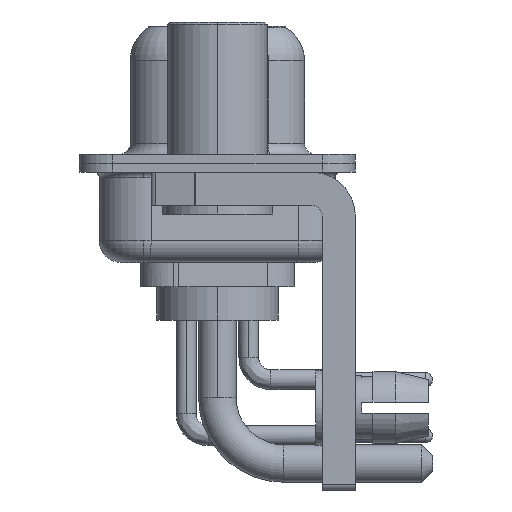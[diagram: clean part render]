
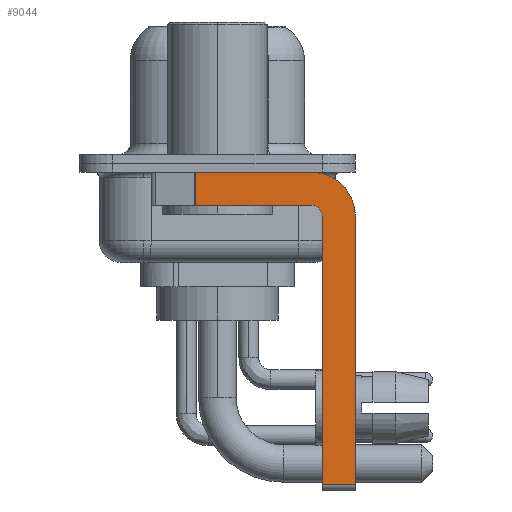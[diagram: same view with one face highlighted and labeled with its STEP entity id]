
A CAD part, left-side view. The second image highlights one B-rep face of the part: STEP entity #9044.
In plain terms, the highlighted planar face has unit normal (-1, 0, 0).
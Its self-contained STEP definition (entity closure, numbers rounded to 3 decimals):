
#429 = CARTESIAN_POINT ( 'NONE',  ( -2.9, 0.978, -0.4 ) ) ;
#444 = LINE ( 'NONE', #2135, #15913 ) ;
#1451 = EDGE_CURVE ( 'NONE', #15932, #14451, #21649, .T. ) ;
#1742 = LINE ( 'NONE', #19196, #20685 ) ;
#1947 = ORIENTED_EDGE ( 'NONE', *, *, #2216, .F. ) ;
#2135 = CARTESIAN_POINT ( 'NONE',  ( -2.9, -4.75, -14.8 ) ) ;
#2216 = EDGE_CURVE ( 'NONE', #13963, #22354, #444, .T. ) ;
#2431 = CARTESIAN_POINT ( 'NONE',  ( -2.9, 3., -0.4 ) ) ;
#3409 = ORIENTED_EDGE ( 'NONE', *, *, #5935, .T. ) ;
#3666 = CARTESIAN_POINT ( 'NONE',  ( -2.9, -4.25, -1.9 ) ) ;
#3979 = DIRECTION ( 'NONE',  ( 0., -1., 0. ) ) ;
#4339 = EDGE_CURVE ( 'NONE', #4758, #15932, #11990, .T. ) ;
#4372 = DIRECTION ( 'NONE',  ( 0., 0., 1. ) ) ;
#4391 = DIRECTION ( 'NONE',  ( 0., -1., 0. ) ) ;
#4398 = ORIENTED_EDGE ( 'NONE', *, *, #11239, .F. ) ;
#4399 = DIRECTION ( 'NONE',  ( 1., 0., 0. ) ) ;
#4554 = CARTESIAN_POINT ( 'NONE',  ( -2.9, 0.978, -1.9 ) ) ;
#4758 = VERTEX_POINT ( 'NONE', #429 ) ;
#5145 = CARTESIAN_POINT ( 'NONE',  ( -2.9, -6.25, -2.4 ) ) ;
#5476 = ORIENTED_EDGE ( 'NONE', *, *, #14808, .F. ) ;
#5899 = CARTESIAN_POINT ( 'NONE',  ( -2.9, 0.978, -1.9 ) ) ;
#5935 = EDGE_CURVE ( 'NONE', #13963, #12385, #1742, .T. ) ;
#6357 = VECTOR ( 'NONE', #11318, 1000. ) ;
#7087 = DIRECTION ( 'NONE',  ( 0., 0., -1. ) ) ;
#7424 = LINE ( 'NONE', #3666, #24733 ) ;
#7636 = AXIS2_PLACEMENT_3D ( 'NONE', #19378, #23122, #13199 ) ;
#7933 = ORIENTED_EDGE ( 'NONE', *, *, #4339, .F. ) ;
#8873 = FACE_OUTER_BOUND ( 'NONE', #24034, .T. ) ;
#9001 = PLANE ( 'NONE',  #21960 ) ;
#9044 = ADVANCED_FACE ( 'NONE', ( #8873 ), #9001, .F. ) ;
#9965 = ORIENTED_EDGE ( 'NONE', *, *, #25151, .F. ) ;
#10228 = EDGE_CURVE ( 'NONE', #4758, #19383, #19434, .T. ) ;
#11208 = CARTESIAN_POINT ( 'NONE',  ( -2.9, -6.25, -14.55 ) ) ;
#11239 = EDGE_CURVE ( 'NONE', #22354, #20326, #18748, .T. ) ;
#11318 = DIRECTION ( 'NONE',  ( 0., 0., -1. ) ) ;
#11990 = LINE ( 'NONE', #2431, #24929 ) ;
#12385 = VERTEX_POINT ( 'NONE', #11208 ) ;
#12394 = ORIENTED_EDGE ( 'NONE', *, *, #1451, .F. ) ;
#12467 = CARTESIAN_POINT ( 'NONE',  ( -2.9, -6.25, -2.4 ) ) ;
#13188 = CARTESIAN_POINT ( 'NONE',  ( -2.9, -4.75, -2.4 ) ) ;
#13199 = DIRECTION ( 'NONE',  ( 0., 0., 1. ) ) ;
#13963 = VERTEX_POINT ( 'NONE', #17521 ) ;
#14451 = VERTEX_POINT ( 'NONE', #12467 ) ;
#14665 = DIRECTION ( 'NONE',  ( 0., 0., -1. ) ) ;
#14808 = EDGE_CURVE ( 'NONE', #20326, #19383, #7424, .T. ) ;
#15913 = VECTOR ( 'NONE', #4372, 1000. ) ;
#15932 = VERTEX_POINT ( 'NONE', #21088 ) ;
#16484 = ORIENTED_EDGE ( 'NONE', *, *, #10228, .T. ) ;
#16702 = DIRECTION ( 'NONE',  ( 1., 0., 0. ) ) ;
#17521 = CARTESIAN_POINT ( 'NONE',  ( -2.9, -4.75, -14.55 ) ) ;
#18748 = CIRCLE ( 'NONE', #7636, 0.5 ) ;
#19196 = CARTESIAN_POINT ( 'NONE',  ( -2.9, -4.25, -14.55 ) ) ;
#19378 = CARTESIAN_POINT ( 'NONE',  ( -2.9, -4.25, -2.4 ) ) ;
#19383 = VERTEX_POINT ( 'NONE', #4554 ) ;
#19434 = LINE ( 'NONE', #5899, #6357 ) ;
#19901 = VECTOR ( 'NONE', #7087, 1000. ) ;
#20326 = VERTEX_POINT ( 'NONE', #20842 ) ;
#20685 = VECTOR ( 'NONE', #3979, 1000. ) ;
#20717 = CARTESIAN_POINT ( 'NONE',  ( -2.9, -4.25, -2.4 ) ) ;
#20842 = CARTESIAN_POINT ( 'NONE',  ( -2.9, -4.25, -1.9 ) ) ;
#21088 = CARTESIAN_POINT ( 'NONE',  ( -2.9, -4.25, -0.4 ) ) ;
#21649 = CIRCLE ( 'NONE', #22478, 2. ) ;
#21960 = AXIS2_PLACEMENT_3D ( 'NONE', #20717, #16702, #14665 ) ;
#22354 = VERTEX_POINT ( 'NONE', #13188 ) ;
#22478 = AXIS2_PLACEMENT_3D ( 'NONE', #24138, #4399, #23756 ) ;
#22949 = LINE ( 'NONE', #5145, #19901 ) ;
#23122 = DIRECTION ( 'NONE',  ( -1., 0., 0. ) ) ;
#23756 = DIRECTION ( 'NONE',  ( 0., 0., -1. ) ) ;
#24034 = EDGE_LOOP ( 'NONE', ( #7933, #16484, #5476, #4398, #1947, #3409, #9965, #12394 ) ) ;
#24138 = CARTESIAN_POINT ( 'NONE',  ( -2.9, -4.25, -2.4 ) ) ;
#24733 = VECTOR ( 'NONE', #25222, 1000. ) ;
#24929 = VECTOR ( 'NONE', #4391, 1000. ) ;
#25151 = EDGE_CURVE ( 'NONE', #14451, #12385, #22949, .T. ) ;
#25222 = DIRECTION ( 'NONE',  ( 0., 1., 0. ) ) ;
